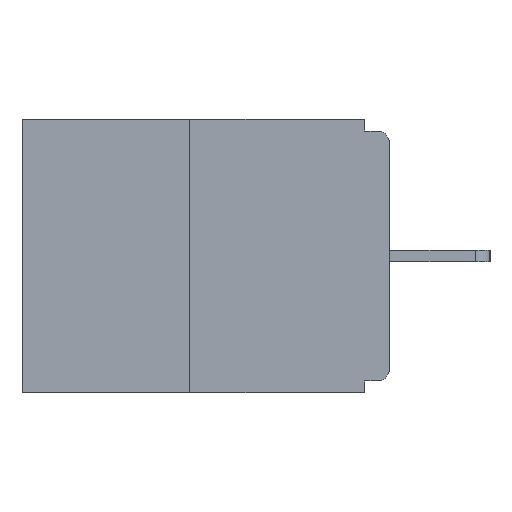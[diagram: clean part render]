
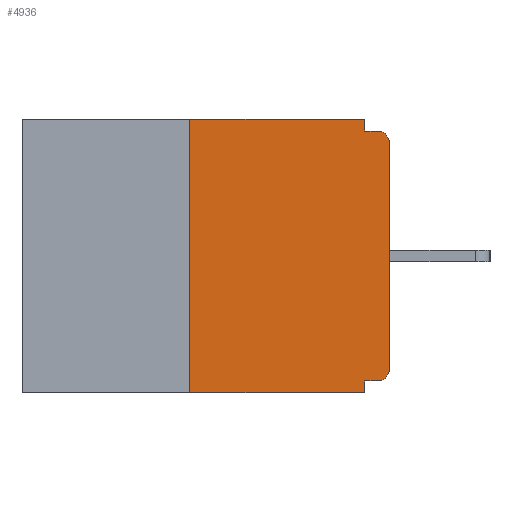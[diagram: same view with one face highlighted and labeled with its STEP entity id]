
A CAD part, left-side view. The second image highlights one B-rep face of the part: STEP entity #4936.
In plain terms, the highlighted planar face has unit normal (-1, 0, 0).
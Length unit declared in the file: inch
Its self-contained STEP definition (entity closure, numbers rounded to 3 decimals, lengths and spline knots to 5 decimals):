
#137 = CARTESIAN_POINT ( 'NONE',  ( 0., 0.031, -0.343 ) ) ;
#196 = ORIENTED_EDGE ( 'NONE', *, *, #3938, .F. ) ;
#298 = VERTEX_POINT ( 'NONE', #5696 ) ;
#532 = AXIS2_PLACEMENT_3D ( 'NONE', #1741, #7499, #6414 ) ;
#784 = ORIENTED_EDGE ( 'NONE', *, *, #4792, .T. ) ;
#823 = CARTESIAN_POINT ( 'NONE',  ( 0., 0., -0.015 ) ) ;
#893 = LINE ( 'NONE', #823, #12591 ) ;
#911 = ORIENTED_EDGE ( 'NONE', *, *, #7875, .F. ) ;
#945 = CARTESIAN_POINT ( 'NONE',  ( 0., 0.25, -0.343 ) ) ;
#1051 = VERTEX_POINT ( 'NONE', #945 ) ;
#1134 = LINE ( 'NONE', #2862, #6165 ) ;
#1182 = DIRECTION ( 'NONE',  ( 0., -1., 0. ) ) ;
#1315 = LINE ( 'NONE', #7923, #11840 ) ;
#1527 = VERTEX_POINT ( 'NONE', #12126 ) ;
#1741 = CARTESIAN_POINT ( 'NONE',  ( 0., 0.46, 0. ) ) ;
#1946 = DIRECTION ( 'NONE',  ( 0., 0., -1. ) ) ;
#1965 = DIRECTION ( 'NONE',  ( 0., 0., -1. ) ) ;
#1974 = DIRECTION ( 'NONE',  ( 0., 0., 1. ) ) ;
#2049 = CARTESIAN_POINT ( 'NONE',  ( 0., 0.46, 0. ) ) ;
#2218 = VERTEX_POINT ( 'NONE', #12015 ) ;
#2225 = CIRCLE ( 'NONE', #7552, 0.015 ) ;
#2369 = CARTESIAN_POINT ( 'NONE',  ( 0., 0.25, 0. ) ) ;
#2862 = CARTESIAN_POINT ( 'NONE',  ( 0., 0.031, 0. ) ) ;
#2947 = LINE ( 'NONE', #6863, #3574 ) ;
#3237 = VECTOR ( 'NONE', #4099, 39.37008 ) ;
#3285 = EDGE_CURVE ( 'NONE', #1051, #5190, #7199, .T. ) ;
#3316 = CARTESIAN_POINT ( 'NONE',  ( 0., 0.25, 0. ) ) ;
#3574 = VECTOR ( 'NONE', #1974, 39.37008 ) ;
#3642 = PLANE ( 'NONE',  #532 ) ;
#3938 = EDGE_CURVE ( 'NONE', #2218, #9774, #893, .T. ) ;
#4099 = DIRECTION ( 'NONE',  ( 0., -1., 0. ) ) ;
#4144 = CARTESIAN_POINT ( 'NONE',  ( 0., 0.015, -0.015 ) ) ;
#4310 = DIRECTION ( 'NONE',  ( 0., 0., -1. ) ) ;
#4493 = DIRECTION ( 'NONE',  ( 0., 0., -1. ) ) ;
#4792 = EDGE_CURVE ( 'NONE', #11800, #298, #2947, .T. ) ;
#4936 = ADVANCED_FACE ( 'NONE', ( #12351 ), #3642, .F. ) ;
#5028 = DIRECTION ( 'NONE',  ( 0., 1., 0. ) ) ;
#5190 = VERTEX_POINT ( 'NONE', #3316 ) ;
#5361 = ORIENTED_EDGE ( 'NONE', *, *, #11116, .F. ) ;
#5696 = CARTESIAN_POINT ( 'NONE',  ( 0., 0., -0.03 ) ) ;
#5899 = LINE ( 'NONE', #2049, #3237 ) ;
#6165 = VECTOR ( 'NONE', #1946, 39.37008 ) ;
#6408 = ORIENTED_EDGE ( 'NONE', *, *, #9244, .F. ) ;
#6414 = DIRECTION ( 'NONE',  ( 0., 0., -1. ) ) ;
#6472 = ORIENTED_EDGE ( 'NONE', *, *, #3285, .F. ) ;
#6485 = LINE ( 'NONE', #11326, #12043 ) ;
#6797 = DIRECTION ( 'NONE',  ( -1., 0., 0. ) ) ;
#6863 = CARTESIAN_POINT ( 'NONE',  ( 0., 0., 0. ) ) ;
#7199 = LINE ( 'NONE', #2369, #10312 ) ;
#7211 = LINE ( 'NONE', #11089, #10039 ) ;
#7231 = EDGE_CURVE ( 'NONE', #9161, #1527, #1315, .T. ) ;
#7255 = DIRECTION ( 'NONE',  ( 0., 0., 1. ) ) ;
#7354 = CIRCLE ( 'NONE', #9593, 0.015 ) ;
#7499 = DIRECTION ( 'NONE',  ( 1., 0., 0. ) ) ;
#7552 = AXIS2_PLACEMENT_3D ( 'NONE', #9285, #8338, #4493 ) ;
#7800 = CARTESIAN_POINT ( 'NONE',  ( 0., 0.031, 0. ) ) ;
#7845 = ORIENTED_EDGE ( 'NONE', *, *, #7941, .T. ) ;
#7875 = EDGE_CURVE ( 'NONE', #1527, #8121, #6485, .T. ) ;
#7923 = CARTESIAN_POINT ( 'NONE',  ( 0., 0., -0.328 ) ) ;
#7941 = EDGE_CURVE ( 'NONE', #298, #9774, #2225, .T. ) ;
#8121 = VERTEX_POINT ( 'NONE', #137 ) ;
#8338 = DIRECTION ( 'NONE',  ( -1., 0., 0. ) ) ;
#8797 = EDGE_LOOP ( 'NONE', ( #6408, #6472, #9869, #911, #10354, #10908, #784, #7845, #196, #5361 ) ) ;
#9161 = VERTEX_POINT ( 'NONE', #11597 ) ;
#9244 = EDGE_CURVE ( 'NONE', #5190, #10074, #5899, .T. ) ;
#9285 = CARTESIAN_POINT ( 'NONE',  ( 0., 0.015, -0.03 ) ) ;
#9593 = AXIS2_PLACEMENT_3D ( 'NONE', #10728, #6797, #1965 ) ;
#9692 = EDGE_CURVE ( 'NONE', #9161, #11800, #7354, .T. ) ;
#9774 = VERTEX_POINT ( 'NONE', #4144 ) ;
#9869 = ORIENTED_EDGE ( 'NONE', *, *, #11659, .T. ) ;
#10039 = VECTOR ( 'NONE', #1182, 39.37008 ) ;
#10074 = VERTEX_POINT ( 'NONE', #7800 ) ;
#10312 = VECTOR ( 'NONE', #7255, 39.37008 ) ;
#10354 = ORIENTED_EDGE ( 'NONE', *, *, #7231, .F. ) ;
#10590 = DIRECTION ( 'NONE',  ( 0., -1., 0. ) ) ;
#10728 = CARTESIAN_POINT ( 'NONE',  ( 0., 0.015, -0.313 ) ) ;
#10908 = ORIENTED_EDGE ( 'NONE', *, *, #9692, .T. ) ;
#11089 = CARTESIAN_POINT ( 'NONE',  ( 0., 0.46, -0.343 ) ) ;
#11116 = EDGE_CURVE ( 'NONE', #10074, #2218, #1134, .T. ) ;
#11326 = CARTESIAN_POINT ( 'NONE',  ( 0., 0.031, -0.343 ) ) ;
#11597 = CARTESIAN_POINT ( 'NONE',  ( 0., 0.015, -0.328 ) ) ;
#11659 = EDGE_CURVE ( 'NONE', #1051, #8121, #7211, .T. ) ;
#11800 = VERTEX_POINT ( 'NONE', #12543 ) ;
#11840 = VECTOR ( 'NONE', #5028, 39.37008 ) ;
#12015 = CARTESIAN_POINT ( 'NONE',  ( 0., 0.031, -0.015 ) ) ;
#12043 = VECTOR ( 'NONE', #4310, 39.37008 ) ;
#12126 = CARTESIAN_POINT ( 'NONE',  ( 0., 0.031, -0.328 ) ) ;
#12351 = FACE_OUTER_BOUND ( 'NONE', #8797, .T. ) ;
#12543 = CARTESIAN_POINT ( 'NONE',  ( 0., 0., -0.313 ) ) ;
#12591 = VECTOR ( 'NONE', #10590, 39.37008 ) ;
